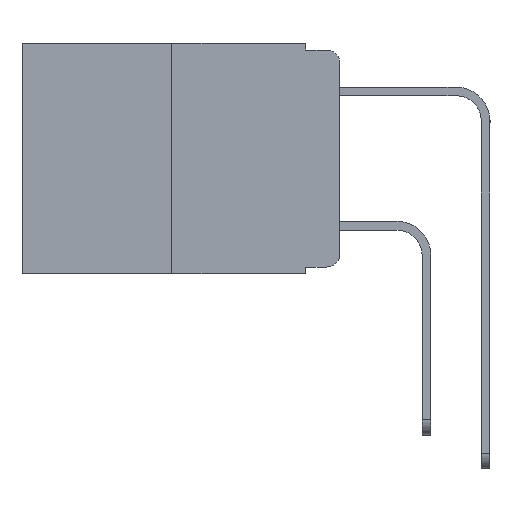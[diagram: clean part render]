
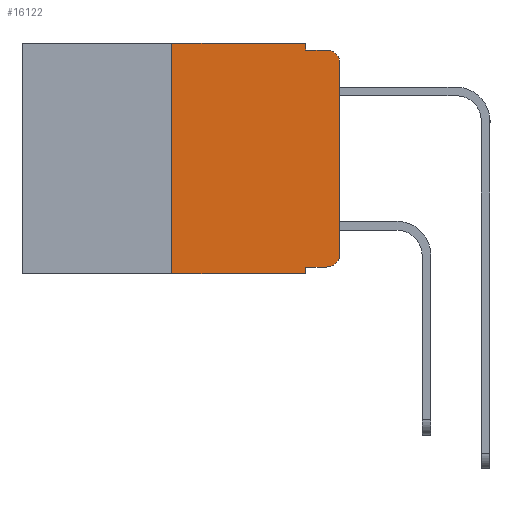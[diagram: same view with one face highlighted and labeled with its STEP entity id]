
A CAD part, left-side view. The second image highlights one B-rep face of the part: STEP entity #16122.
In plain terms, the highlighted planar face has unit normal (-1, 0, 0).
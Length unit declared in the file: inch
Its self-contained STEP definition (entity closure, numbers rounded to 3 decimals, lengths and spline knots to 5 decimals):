
#220 = EDGE_CURVE ( 'NONE', #5174, #18759, #16449, .T. ) ;
#282 = LINE ( 'NONE', #22640, #26257 ) ;
#678 = VECTOR ( 'NONE', #12555, 39.37008 ) ;
#1299 = VERTEX_POINT ( 'NONE', #9659 ) ;
#1397 = CARTESIAN_POINT ( 'NONE',  ( 0., 0.02, -0.03 ) ) ;
#1418 = ORIENTED_EDGE ( 'NONE', *, *, #21952, .T. ) ;
#2628 = EDGE_CURVE ( 'NONE', #3040, #24351, #282, .T. ) ;
#2753 = VERTEX_POINT ( 'NONE', #21141 ) ;
#3040 = VERTEX_POINT ( 'NONE', #14208 ) ;
#3478 = DIRECTION ( 'NONE',  ( 0., 0., -1. ) ) ;
#3900 = AXIS2_PLACEMENT_3D ( 'NONE', #5992, #20442, #8103 ) ;
#4194 = EDGE_CURVE ( 'NONE', #26529, #22385, #6634, .T. ) ;
#4454 = VERTEX_POINT ( 'NONE', #16572 ) ;
#5020 = AXIS2_PLACEMENT_3D ( 'NONE', #1397, #15912, #3478 ) ;
#5051 = CARTESIAN_POINT ( 'NONE',  ( 0., 0., -0.03 ) ) ;
#5174 = VERTEX_POINT ( 'NONE', #13873 ) ;
#5446 = CARTESIAN_POINT ( 'NONE',  ( 0., 0.051, -0.343 ) ) ;
#5603 = ORIENTED_EDGE ( 'NONE', *, *, #2628, .T. ) ;
#5992 = CARTESIAN_POINT ( 'NONE',  ( 0., 0.02, -0.313 ) ) ;
#6634 = LINE ( 'NONE', #21766, #23024 ) ;
#8103 = DIRECTION ( 'NONE',  ( 0., 0., -1. ) ) ;
#8333 = CARTESIAN_POINT ( 'NONE',  ( 0., 0.473, 0. ) ) ;
#8380 = VECTOR ( 'NONE', #17546, 39.37008 ) ;
#8852 = ORIENTED_EDGE ( 'NONE', *, *, #22070, .T. ) ;
#8988 = LINE ( 'NONE', #12004, #24679 ) ;
#9488 = DIRECTION ( 'NONE',  ( 0., 0., -1. ) ) ;
#9500 = ORIENTED_EDGE ( 'NONE', *, *, #12905, .F. ) ;
#9659 = CARTESIAN_POINT ( 'NONE',  ( 0., 0.25, -0.343 ) ) ;
#10415 = DIRECTION ( 'NONE',  ( 0., -1., 0. ) ) ;
#10456 = CARTESIAN_POINT ( 'NONE',  ( 0., 0.473, -0.343 ) ) ;
#10483 = DIRECTION ( 'NONE',  ( 0., 0., -1. ) ) ;
#11609 = CARTESIAN_POINT ( 'NONE',  ( 0., 0.051, -0.01 ) ) ;
#11697 = LINE ( 'NONE', #10456, #678 ) ;
#12004 = CARTESIAN_POINT ( 'NONE',  ( 0., 0.051, 0. ) ) ;
#12555 = DIRECTION ( 'NONE',  ( 0., -1., 0. ) ) ;
#12754 = ORIENTED_EDGE ( 'NONE', *, *, #23482, .F. ) ;
#12905 = EDGE_CURVE ( 'NONE', #3040, #18246, #8988, .T. ) ;
#13405 = CARTESIAN_POINT ( 'NONE',  ( 0., 0.25, 0. ) ) ;
#13873 = CARTESIAN_POINT ( 'NONE',  ( 0., 0., -0.313 ) ) ;
#13961 = CARTESIAN_POINT ( 'NONE',  ( 0., 0., 0. ) ) ;
#14039 = ORIENTED_EDGE ( 'NONE', *, *, #14975, .F. ) ;
#14182 = CARTESIAN_POINT ( 'NONE',  ( 0., 0.02, -0.333 ) ) ;
#14208 = CARTESIAN_POINT ( 'NONE',  ( 0., 0.051, -0.333 ) ) ;
#14584 = CARTESIAN_POINT ( 'NONE',  ( 0., 0.473, 0. ) ) ;
#14975 = EDGE_CURVE ( 'NONE', #22385, #4454, #16596, .T. ) ;
#15326 = ORIENTED_EDGE ( 'NONE', *, *, #4194, .F. ) ;
#15912 = DIRECTION ( 'NONE',  ( -1., 0., 0. ) ) ;
#16122 = ADVANCED_FACE ( 'NONE', ( #21566 ), #20729, .F. ) ;
#16192 = LINE ( 'NONE', #8333, #26283 ) ;
#16449 = LINE ( 'NONE', #13961, #17079 ) ;
#16572 = CARTESIAN_POINT ( 'NONE',  ( 0., 0.02, -0.01 ) ) ;
#16596 = LINE ( 'NONE', #20865, #21320 ) ;
#16883 = DIRECTION ( 'NONE',  ( 0., -1., 0. ) ) ;
#17079 = VECTOR ( 'NONE', #23675, 39.37008 ) ;
#17546 = DIRECTION ( 'NONE',  ( 0., 0., 1. ) ) ;
#18246 = VERTEX_POINT ( 'NONE', #5446 ) ;
#18249 = EDGE_CURVE ( 'NONE', #18759, #4454, #19615, .T. ) ;
#18616 = DIRECTION ( 'NONE',  ( 0., -1., 0. ) ) ;
#18759 = VERTEX_POINT ( 'NONE', #5051 ) ;
#19140 = CIRCLE ( 'NONE', #3900, 0.02 ) ;
#19498 = CARTESIAN_POINT ( 'NONE',  ( 0., 0.051, 0. ) ) ;
#19615 = CIRCLE ( 'NONE', #5020, 0.02 ) ;
#20442 = DIRECTION ( 'NONE',  ( -1., 0., 0. ) ) ;
#20729 = PLANE ( 'NONE',  #21561 ) ;
#20865 = CARTESIAN_POINT ( 'NONE',  ( 0., 0.051, -0.01 ) ) ;
#21034 = ORIENTED_EDGE ( 'NONE', *, *, #18249, .T. ) ;
#21141 = CARTESIAN_POINT ( 'NONE',  ( 0., 0.25, 0. ) ) ;
#21320 = VECTOR ( 'NONE', #16883, 39.37008 ) ;
#21561 = AXIS2_PLACEMENT_3D ( 'NONE', #14584, #22738, #10483 ) ;
#21566 = FACE_OUTER_BOUND ( 'NONE', #22276, .T. ) ;
#21766 = CARTESIAN_POINT ( 'NONE',  ( 0., 0.051, 0. ) ) ;
#21952 = EDGE_CURVE ( 'NONE', #24351, #5174, #19140, .T. ) ;
#22070 = EDGE_CURVE ( 'NONE', #1299, #18246, #11697, .T. ) ;
#22260 = DIRECTION ( 'NONE',  ( 0., 0., -1. ) ) ;
#22276 = EDGE_LOOP ( 'NONE', ( #25122, #21034, #14039, #15326, #23886, #12754, #8852, #9500, #5603, #1418 ) ) ;
#22385 = VERTEX_POINT ( 'NONE', #11609 ) ;
#22640 = CARTESIAN_POINT ( 'NONE',  ( 0., 0.051, -0.333 ) ) ;
#22738 = DIRECTION ( 'NONE',  ( 1., 0., 0. ) ) ;
#23024 = VECTOR ( 'NONE', #9488, 39.37008 ) ;
#23166 = EDGE_CURVE ( 'NONE', #2753, #26529, #16192, .T. ) ;
#23482 = EDGE_CURVE ( 'NONE', #1299, #2753, #25335, .T. ) ;
#23675 = DIRECTION ( 'NONE',  ( 0., 0., 1. ) ) ;
#23886 = ORIENTED_EDGE ( 'NONE', *, *, #23166, .F. ) ;
#24351 = VERTEX_POINT ( 'NONE', #14182 ) ;
#24679 = VECTOR ( 'NONE', #22260, 39.37008 ) ;
#25122 = ORIENTED_EDGE ( 'NONE', *, *, #220, .T. ) ;
#25335 = LINE ( 'NONE', #13405, #8380 ) ;
#26257 = VECTOR ( 'NONE', #18616, 39.37008 ) ;
#26283 = VECTOR ( 'NONE', #10415, 39.37008 ) ;
#26529 = VERTEX_POINT ( 'NONE', #19498 ) ;
